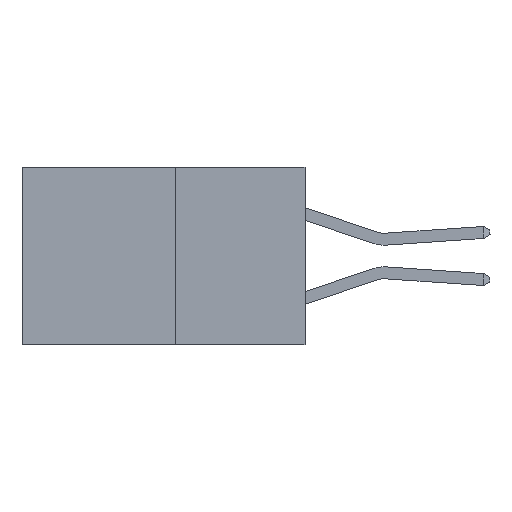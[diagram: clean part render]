
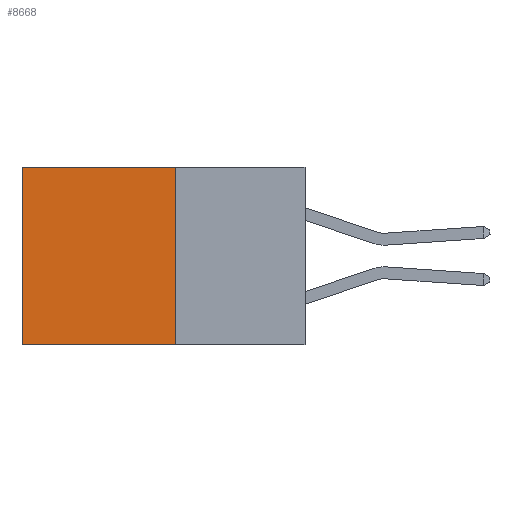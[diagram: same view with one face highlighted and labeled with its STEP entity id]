
A CAD part, left-side view. The second image highlights one B-rep face of the part: STEP entity #8668.
In plain terms, the highlighted planar face has unit normal (-1, 0, 0).
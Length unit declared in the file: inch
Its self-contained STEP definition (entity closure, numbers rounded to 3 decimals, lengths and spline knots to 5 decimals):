
#712 = VERTEX_POINT ( 'NONE', #840 ) ;
#840 = CARTESIAN_POINT ( 'NONE',  ( 0.277, 0.27, 0. ) ) ;
#884 = CARTESIAN_POINT ( 'NONE',  ( 0.277, 0.59, 0. ) ) ;
#1331 = CARTESIAN_POINT ( 'NONE',  ( 0.277, 0.59, -0.37 ) ) ;
#1851 = CARTESIAN_POINT ( 'NONE',  ( 0.277, 0.27, -0.37 ) ) ;
#3310 = PLANE ( 'NONE',  #13945 ) ;
#4086 = ORIENTED_EDGE ( 'NONE', *, *, #7323, .F. ) ;
#4482 = ORIENTED_EDGE ( 'NONE', *, *, #7055, .T. ) ;
#4710 = DIRECTION ( 'NONE',  ( 0., 0., -1. ) ) ;
#5166 = VECTOR ( 'NONE', #9108, 39.37008 ) ;
#5458 = DIRECTION ( 'NONE',  ( 0., 0., -1. ) ) ;
#5462 = EDGE_CURVE ( 'NONE', #7936, #16312, #12675, .T. ) ;
#6365 = CARTESIAN_POINT ( 'NONE',  ( 0.277, 0.27, 0. ) ) ;
#7055 = EDGE_CURVE ( 'NONE', #15900, #16312, #7488, .T. ) ;
#7323 = EDGE_CURVE ( 'NONE', #712, #7936, #15343, .T. ) ;
#7488 = LINE ( 'NONE', #1331, #14269 ) ;
#7936 = VERTEX_POINT ( 'NONE', #1851 ) ;
#8062 = ORIENTED_EDGE ( 'NONE', *, *, #5462, .F. ) ;
#8196 = VECTOR ( 'NONE', #8597, 39.37008 ) ;
#8597 = DIRECTION ( 'NONE',  ( 0., 0., -1. ) ) ;
#8668 = ADVANCED_FACE ( 'NONE', ( #12431 ), #3310, .F. ) ;
#8819 = ORIENTED_EDGE ( 'NONE', *, *, #11444, .T. ) ;
#9108 = DIRECTION ( 'NONE',  ( 0., 1., 0. ) ) ;
#9870 = EDGE_LOOP ( 'NONE', ( #4482, #8062, #4086, #8819 ) ) ;
#9959 = DIRECTION ( 'NONE',  ( 0., 1., 0. ) ) ;
#10060 = CARTESIAN_POINT ( 'NONE',  ( 0.277, 0.27, -0.37 ) ) ;
#10179 = CARTESIAN_POINT ( 'NONE',  ( 0.277, 0.59, -0.37 ) ) ;
#11444 = EDGE_CURVE ( 'NONE', #712, #15900, #15844, .T. ) ;
#12431 = FACE_OUTER_BOUND ( 'NONE', #9870, .T. ) ;
#12675 = LINE ( 'NONE', #16577, #16156 ) ;
#12790 = DIRECTION ( 'NONE',  ( 1., 0., 0. ) ) ;
#13945 = AXIS2_PLACEMENT_3D ( 'NONE', #10060, #12790, #4710 ) ;
#13980 = CARTESIAN_POINT ( 'NONE',  ( 0.277, 0.27, -0.37 ) ) ;
#14269 = VECTOR ( 'NONE', #5458, 39.37008 ) ;
#15343 = LINE ( 'NONE', #13980, #8196 ) ;
#15844 = LINE ( 'NONE', #6365, #5166 ) ;
#15900 = VERTEX_POINT ( 'NONE', #884 ) ;
#16156 = VECTOR ( 'NONE', #9959, 39.37008 ) ;
#16312 = VERTEX_POINT ( 'NONE', #10179 ) ;
#16577 = CARTESIAN_POINT ( 'NONE',  ( 0.277, 0.27, -0.37 ) ) ;
